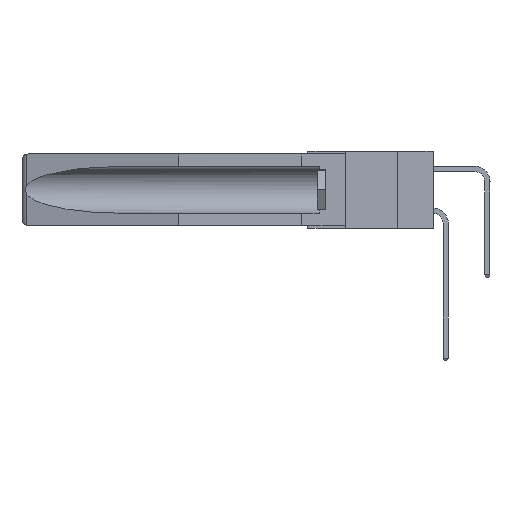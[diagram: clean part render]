
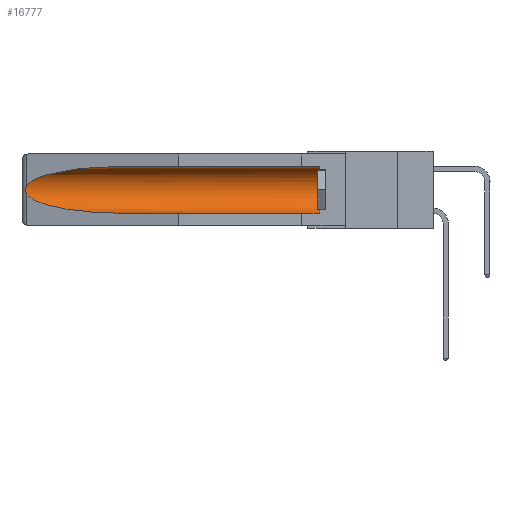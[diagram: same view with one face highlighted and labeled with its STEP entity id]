
A CAD part, left-side view. The second image highlights one B-rep face of the part: STEP entity #16777.
In plain terms, the highlighted cylindrical face has radius 2.857 mm (diameter 5.715 mm), a partial arc.
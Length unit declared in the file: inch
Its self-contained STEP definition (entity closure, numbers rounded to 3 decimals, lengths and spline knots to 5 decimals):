
#78 = VERTEX_POINT ( 'NONE', #19647 ) ;
#664 = CARTESIAN_POINT ( 'NONE',  ( 0.26597, 1.52961, -0.15275 ) ) ;
#807 = CARTESIAN_POINT ( 'NONE',  ( 0.26655, 1.53094, -0.18657 ) ) ;
#957 = CARTESIAN_POINT ( 'NONE',  ( 0.2673, 1.5327, -0.16383 ) ) ;
#2457 = ORIENTED_EDGE ( 'NONE', *, *, #5929, .T. ) ;
#2738 = CARTESIAN_POINT ( 'NONE',  ( 0.2673, 1.53269, -0.17917 ) ) ;
#3232 = VECTOR ( 'NONE', #20759, 39.37008 ) ;
#3487 = AXIS2_PLACEMENT_3D ( 'NONE', #10352, #22627, #15571 ) ;
#3563 = CARTESIAN_POINT ( 'NONE',  ( 0.26537, 1.52718, -0.19328 ) ) ;
#3898 = CARTESIAN_POINT ( 'NONE',  ( 0.155, -0.30754, -0.1715 ) ) ;
#4058 = DIRECTION ( 'NONE',  ( 0., 1., 0. ) ) ;
#4449 = CARTESIAN_POINT ( 'NONE',  ( 0.26654, 1.53092, -0.15636 ) ) ;
#4789 = LINE ( 'NONE', #10518, #13572 ) ;
#5182 = EDGE_CURVE ( 'NONE', #17593, #18588, #20992, .T. ) ;
#5463 = LINE ( 'NONE', #15611, #3232 ) ;
#5929 = EDGE_CURVE ( 'NONE', #19367, #78, #14269, .T. ) ;
#6053 = EDGE_CURVE ( 'NONE', #78, #8074, #13299, .T. ) ;
#6725 = CARTESIAN_POINT ( 'NONE',  ( 0.155, 1.07973, -0.059 ) ) ;
#7149 = ORIENTED_EDGE ( 'NONE', *, *, #6053, .T. ) ;
#7332 = CYLINDRICAL_SURFACE ( 'NONE', #13855, 0.1125 ) ;
#7508 = VERTEX_POINT ( 'NONE', #15904 ) ;
#8074 = VERTEX_POINT ( 'NONE', #3563 ) ;
#8535 = CARTESIAN_POINT ( 'NONE',  ( 0.155, 1.07973, -0.284 ) ) ;
#9010 = ORIENTED_EDGE ( 'NONE', *, *, #11102, .T. ) ;
#9219 =( BOUNDED_CURVE ( )  B_SPLINE_CURVE ( 3, ( #17188, #13611, #15438, #8535 ),
 .UNSPECIFIED., .F., .F. ) 
 B_SPLINE_CURVE_WITH_KNOTS ( ( 4, 4 ),
 ( 0.1948, 1.5708 ),
 .UNSPECIFIED. ) 
 CURVE ( )  GEOMETRIC_REPRESENTATION_ITEM ( )  RATIONAL_B_SPLINE_CURVE ( ( 1., 0.848, 0.848, 1. ) ) 
 REPRESENTATION_ITEM ( '' )  );
#9660 = CARTESIAN_POINT ( 'NONE',  ( 0.2675, 1.53308, -0.16763 ) ) ;
#10352 = CARTESIAN_POINT ( 'NONE',  ( 0.155, 0.126, -0.1715 ) ) ;
#10518 = CARTESIAN_POINT ( 'NONE',  ( 0.155, -0.30754, -0.284 ) ) ;
#11102 = EDGE_CURVE ( 'NONE', #18588, #19367, #5463, .T. ) ;
#11910 = CARTESIAN_POINT ( 'NONE',  ( 0.25451, 1.48313, -0.09465 ) ) ;
#11914 = CARTESIAN_POINT ( 'NONE',  ( 0.155, 1.07973, -0.059 ) ) ;
#12135 = CARTESIAN_POINT ( 'NONE',  ( 0.26537, 1.52718, -0.14972 ) ) ;
#12856 = CARTESIAN_POINT ( 'NONE',  ( 0.155, 0.126, -0.059 ) ) ;
#13029 = ORIENTED_EDGE ( 'NONE', *, *, #19395, .T. ) ;
#13299 = B_SPLINE_CURVE_WITH_KNOTS ( 'NONE', 3,
 ( #18470, #664, #4449, #957, #9660, #16626, #2738, #807, #20252, #21929 ),
 .UNSPECIFIED., .F., .F.,
 ( 4, 2, 2, 2, 4 ),
 ( 0., 0.00029, 0.00058, 0.00087, 0.00117 ),
 .UNSPECIFIED. ) ;
#13572 = VECTOR ( 'NONE', #14278, 39.37008 ) ;
#13611 = CARTESIAN_POINT ( 'NONE',  ( 0.25451, 1.48313, -0.24835 ) ) ;
#13855 = AXIS2_PLACEMENT_3D ( 'NONE', #3898, #4058, #19709 ) ;
#14269 =( BOUNDED_CURVE ( )  B_SPLINE_CURVE ( 3, ( #6725, #22638, #11910, #12135 ),
 .UNSPECIFIED., .F., .F. ) 
 B_SPLINE_CURVE_WITH_KNOTS ( ( 4, 4 ),
 ( 4.71239, 6.08839 ),
 .UNSPECIFIED. ) 
 CURVE ( )  GEOMETRIC_REPRESENTATION_ITEM ( )  RATIONAL_B_SPLINE_CURVE ( ( 1., 0.848, 0.848, 1. ) ) 
 REPRESENTATION_ITEM ( '' )  );
#14278 = DIRECTION ( 'NONE',  ( 0., 1., 0. ) ) ;
#15438 = CARTESIAN_POINT ( 'NONE',  ( 0.21114, 1.30732, -0.284 ) ) ;
#15571 = DIRECTION ( 'NONE',  ( 0., 0., 1. ) ) ;
#15611 = CARTESIAN_POINT ( 'NONE',  ( 0.155, -0.30754, -0.059 ) ) ;
#15721 = EDGE_LOOP ( 'NONE', ( #2457, #7149, #13029, #16290, #17316, #9010 ) ) ;
#15904 = CARTESIAN_POINT ( 'NONE',  ( 0.155, 1.07973, -0.284 ) ) ;
#16290 = ORIENTED_EDGE ( 'NONE', *, *, #19491, .F. ) ;
#16626 = CARTESIAN_POINT ( 'NONE',  ( 0.2675, 1.53308, -0.17534 ) ) ;
#16777 = ADVANCED_FACE ( 'NONE', ( #17184 ), #7332, .F. ) ;
#16930 = CARTESIAN_POINT ( 'NONE',  ( 0.155, 0.126, -0.284 ) ) ;
#17184 = FACE_OUTER_BOUND ( 'NONE', #15721, .T. ) ;
#17188 = CARTESIAN_POINT ( 'NONE',  ( 0.26537, 1.52718, -0.19328 ) ) ;
#17316 = ORIENTED_EDGE ( 'NONE', *, *, #5182, .T. ) ;
#17593 = VERTEX_POINT ( 'NONE', #16930 ) ;
#18470 = CARTESIAN_POINT ( 'NONE',  ( 0.26537, 1.52718, -0.14972 ) ) ;
#18588 = VERTEX_POINT ( 'NONE', #12856 ) ;
#19367 = VERTEX_POINT ( 'NONE', #11914 ) ;
#19395 = EDGE_CURVE ( 'NONE', #8074, #7508, #9219, .T. ) ;
#19491 = EDGE_CURVE ( 'NONE', #17593, #7508, #4789, .T. ) ;
#19647 = CARTESIAN_POINT ( 'NONE',  ( 0.26537, 1.52718, -0.14972 ) ) ;
#19709 = DIRECTION ( 'NONE',  ( 0., 0., 1. ) ) ;
#20252 = CARTESIAN_POINT ( 'NONE',  ( 0.26597, 1.5296, -0.19026 ) ) ;
#20759 = DIRECTION ( 'NONE',  ( 0., 1., 0. ) ) ;
#20992 = CIRCLE ( 'NONE', #3487, 0.1125 ) ;
#21929 = CARTESIAN_POINT ( 'NONE',  ( 0.26537, 1.52718, -0.19328 ) ) ;
#22627 = DIRECTION ( 'NONE',  ( 0., -1., 0. ) ) ;
#22638 = CARTESIAN_POINT ( 'NONE',  ( 0.21114, 1.30732, -0.059 ) ) ;
